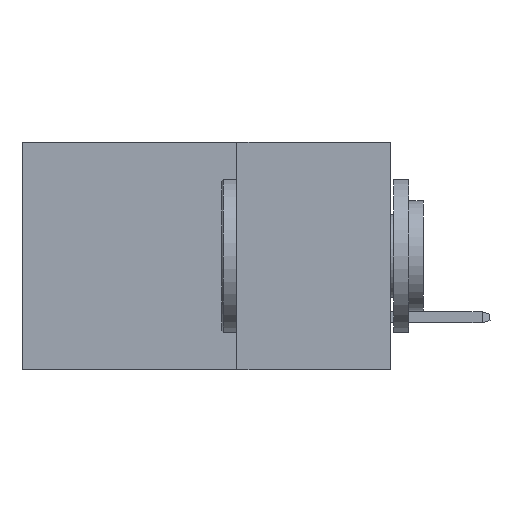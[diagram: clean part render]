
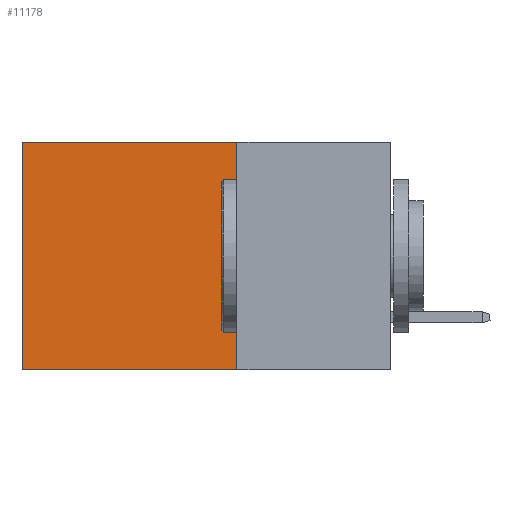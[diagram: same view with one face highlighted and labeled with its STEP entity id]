
A CAD part, left-side view. The second image highlights one B-rep face of the part: STEP entity #11178.
In plain terms, the highlighted planar face has unit normal (-1, 0, 0).
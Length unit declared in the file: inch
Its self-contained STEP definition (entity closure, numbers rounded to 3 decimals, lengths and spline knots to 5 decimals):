
#23 = ORIENTED_EDGE ( 'NONE', *, *, #8441, .F. ) ;
#189 = DIRECTION ( 'NONE',  ( 1., 0., 0. ) ) ;
#421 = VECTOR ( 'NONE', #3739, 39.37008 ) ;
#1098 = VERTEX_POINT ( 'NONE', #7486 ) ;
#1249 = VERTEX_POINT ( 'NONE', #6392 ) ;
#1655 = VERTEX_POINT ( 'NONE', #5833 ) ;
#1748 = ORIENTED_EDGE ( 'NONE', *, *, #11228, .T. ) ;
#2281 = VERTEX_POINT ( 'NONE', #6097 ) ;
#2446 = EDGE_CURVE ( 'NONE', #1098, #1249, #2603, .T. ) ;
#2507 = VECTOR ( 'NONE', #7850, 39.37008 ) ;
#2603 = LINE ( 'NONE', #2803, #4055 ) ;
#2803 = CARTESIAN_POINT ( 'NONE',  ( 0.2875, 0.25, 0. ) ) ;
#3485 = LINE ( 'NONE', #5893, #2507 ) ;
#3739 = DIRECTION ( 'NONE',  ( 0., 1., 0. ) ) ;
#4055 = VECTOR ( 'NONE', #4886, 39.37008 ) ;
#4886 = DIRECTION ( 'NONE',  ( 0., 0., -1. ) ) ;
#5833 = CARTESIAN_POINT ( 'NONE',  ( 0.2875, 0.6, -0.37 ) ) ;
#5893 = CARTESIAN_POINT ( 'NONE',  ( 0.2875, 0.6, 0. ) ) ;
#6097 = CARTESIAN_POINT ( 'NONE',  ( 0.2875, 0.6, 0. ) ) ;
#6392 = CARTESIAN_POINT ( 'NONE',  ( 0.2875, 0.25, -0.37 ) ) ;
#6491 = EDGE_CURVE ( 'NONE', #2281, #1655, #3485, .T. ) ;
#6741 = ORIENTED_EDGE ( 'NONE', *, *, #6491, .T. ) ;
#7294 = PLANE ( 'NONE',  #9675 ) ;
#7342 = DIRECTION ( 'NONE',  ( 0., 0., -1. ) ) ;
#7486 = CARTESIAN_POINT ( 'NONE',  ( 0.2875, 0.25, 0. ) ) ;
#7850 = DIRECTION ( 'NONE',  ( 0., 0., -1. ) ) ;
#8325 = CARTESIAN_POINT ( 'NONE',  ( 0.2875, 0.25, 0. ) ) ;
#8335 = LINE ( 'NONE', #11449, #11798 ) ;
#8441 = EDGE_CURVE ( 'NONE', #1249, #1655, #10427, .T. ) ;
#9675 = AXIS2_PLACEMENT_3D ( 'NONE', #8325, #189, #7342 ) ;
#9834 = CARTESIAN_POINT ( 'NONE',  ( 0.2875, 0.25, -0.37 ) ) ;
#10028 = EDGE_LOOP ( 'NONE', ( #6741, #23, #11641, #1748 ) ) ;
#10427 = LINE ( 'NONE', #9834, #421 ) ;
#11178 = ADVANCED_FACE ( 'NONE', ( #11330 ), #7294, .F. ) ;
#11228 = EDGE_CURVE ( 'NONE', #1098, #2281, #8335, .T. ) ;
#11330 = FACE_OUTER_BOUND ( 'NONE', #10028, .T. ) ;
#11449 = CARTESIAN_POINT ( 'NONE',  ( 0.2875, 0.25, 0. ) ) ;
#11641 = ORIENTED_EDGE ( 'NONE', *, *, #2446, .F. ) ;
#11798 = VECTOR ( 'NONE', #12603, 39.37008 ) ;
#12603 = DIRECTION ( 'NONE',  ( 0., 1., 0. ) ) ;
